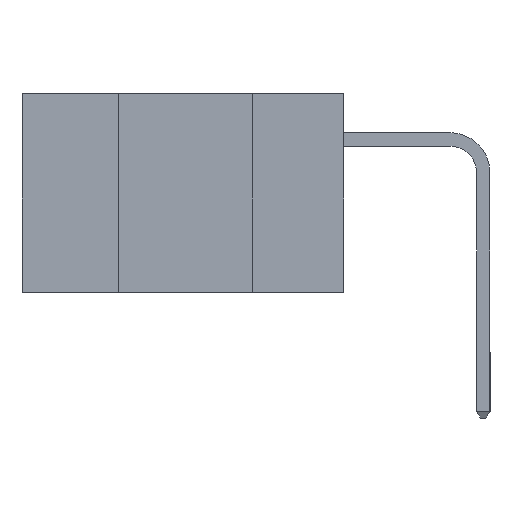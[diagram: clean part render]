
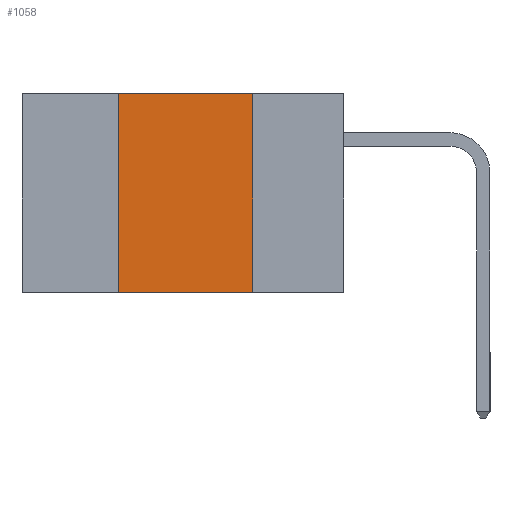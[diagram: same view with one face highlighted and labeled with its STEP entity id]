
A CAD part, left-side view. The second image highlights one B-rep face of the part: STEP entity #1058.
In plain terms, the highlighted planar face has unit normal (-1, 0, 0).
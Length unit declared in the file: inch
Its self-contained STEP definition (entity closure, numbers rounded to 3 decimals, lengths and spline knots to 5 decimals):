
#368 = LINE ( 'NONE', #19838, #1232 ) ;
#1058 = ADVANCED_FACE ( 'NONE', ( #13620 ), #21601, .F. ) ;
#1232 = VECTOR ( 'NONE', #17959, 39.37008 ) ;
#2227 = LINE ( 'NONE', #12958, #5373 ) ;
#2486 = VECTOR ( 'NONE', #9696, 39.37008 ) ;
#3430 = EDGE_CURVE ( 'NONE', #23011, #9018, #4725, .T. ) ;
#4725 = LINE ( 'NONE', #17154, #18415 ) ;
#5283 = CARTESIAN_POINT ( 'NONE',  ( 0., 0.17, 0. ) ) ;
#5373 = VECTOR ( 'NONE', #20667, 39.37008 ) ;
#5509 = EDGE_CURVE ( 'NONE', #14894, #9018, #8587, .T. ) ;
#6821 = DIRECTION ( 'NONE',  ( 1., 0., 0. ) ) ;
#7426 = CARTESIAN_POINT ( 'NONE',  ( 0., 0.42, 0. ) ) ;
#8241 = AXIS2_PLACEMENT_3D ( 'NONE', #17971, #6821, #11142 ) ;
#8587 = LINE ( 'NONE', #20734, #2486 ) ;
#9018 = VERTEX_POINT ( 'NONE', #19650 ) ;
#9696 = DIRECTION ( 'NONE',  ( 0., -1., 0. ) ) ;
#9762 = DIRECTION ( 'NONE',  ( 0., 0., -1. ) ) ;
#11142 = DIRECTION ( 'NONE',  ( 0., 0., -1. ) ) ;
#12757 = ORIENTED_EDGE ( 'NONE', *, *, #3430, .F. ) ;
#12958 = CARTESIAN_POINT ( 'NONE',  ( 0., 0.42, 0. ) ) ;
#13167 = ORIENTED_EDGE ( 'NONE', *, *, #5509, .T. ) ;
#13620 = FACE_OUTER_BOUND ( 'NONE', #15897, .T. ) ;
#14894 = VERTEX_POINT ( 'NONE', #22062 ) ;
#15897 = EDGE_LOOP ( 'NONE', ( #12757, #16019, #20812, #13167 ) ) ;
#16019 = ORIENTED_EDGE ( 'NONE', *, *, #19583, .F. ) ;
#17055 = EDGE_CURVE ( 'NONE', #14894, #23174, #2227, .T. ) ;
#17154 = CARTESIAN_POINT ( 'NONE',  ( 0., 0.17, 0. ) ) ;
#17959 = DIRECTION ( 'NONE',  ( 0., -1., 0. ) ) ;
#17971 = CARTESIAN_POINT ( 'NONE',  ( 0., 0.6, 0. ) ) ;
#18415 = VECTOR ( 'NONE', #9762, 39.37008 ) ;
#19583 = EDGE_CURVE ( 'NONE', #23174, #23011, #368, .T. ) ;
#19650 = CARTESIAN_POINT ( 'NONE',  ( 0., 0.17, -0.37 ) ) ;
#19838 = CARTESIAN_POINT ( 'NONE',  ( 0., 0.6, 0. ) ) ;
#20667 = DIRECTION ( 'NONE',  ( 0., 0., 1. ) ) ;
#20734 = CARTESIAN_POINT ( 'NONE',  ( 0., 0.6, -0.37 ) ) ;
#20812 = ORIENTED_EDGE ( 'NONE', *, *, #17055, .F. ) ;
#21601 = PLANE ( 'NONE',  #8241 ) ;
#22062 = CARTESIAN_POINT ( 'NONE',  ( 0., 0.42, -0.37 ) ) ;
#23011 = VERTEX_POINT ( 'NONE', #5283 ) ;
#23174 = VERTEX_POINT ( 'NONE', #7426 ) ;
